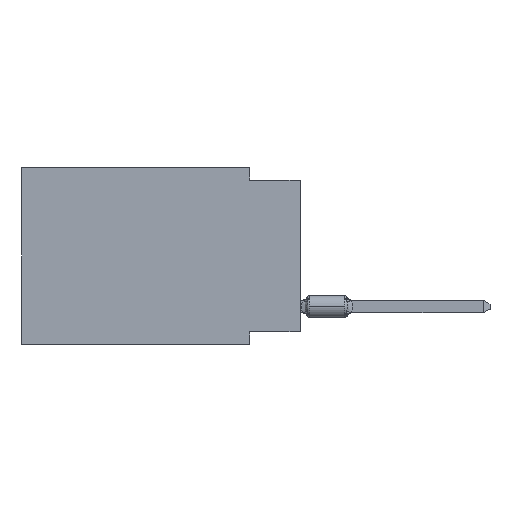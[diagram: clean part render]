
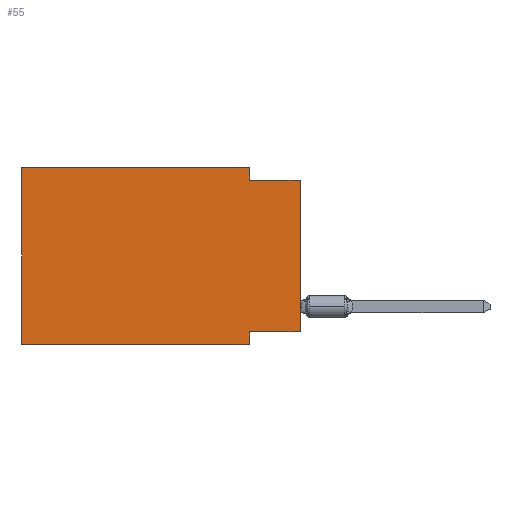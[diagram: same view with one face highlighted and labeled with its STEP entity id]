
A CAD part, left-side view. The second image highlights one B-rep face of the part: STEP entity #55.
In plain terms, the highlighted planar face has unit normal (-1, 0, 0).
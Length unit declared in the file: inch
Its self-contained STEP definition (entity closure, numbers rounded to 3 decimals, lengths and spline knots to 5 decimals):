
#55 = ADVANCED_FACE ( 'NONE', ( #3599 ), #19217, .F. ) ;
#631 = CARTESIAN_POINT ( 'NONE',  ( 0., 0., -0.025 ) ) ;
#648 = EDGE_CURVE ( 'NONE', #3919, #10364, #12601, .T. ) ;
#726 = CARTESIAN_POINT ( 'NONE',  ( 0., 0.1, -0.35 ) ) ;
#1348 = ORIENTED_EDGE ( 'NONE', *, *, #17111, .F. ) ;
#1421 = EDGE_CURVE ( 'NONE', #20242, #12905, #19560, .T. ) ;
#1776 = DIRECTION ( 'NONE',  ( 0., 0., -1. ) ) ;
#1805 = DIRECTION ( 'NONE',  ( 0., 0., 1. ) ) ;
#1895 = EDGE_CURVE ( 'NONE', #14072, #14090, #8160, .T. ) ;
#2567 = DIRECTION ( 'NONE',  ( 0., 1., 0. ) ) ;
#2668 = VECTOR ( 'NONE', #4640, 39.37008 ) ;
#2673 = VECTOR ( 'NONE', #1805, 39.37008 ) ;
#2706 = ORIENTED_EDGE ( 'NONE', *, *, #9855, .F. ) ;
#2844 = CARTESIAN_POINT ( 'NONE',  ( 0., 0.1, 0. ) ) ;
#2940 = DIRECTION ( 'NONE',  ( 0., 0., 1. ) ) ;
#3489 = CARTESIAN_POINT ( 'NONE',  ( 0., 0.1, 0. ) ) ;
#3599 = FACE_OUTER_BOUND ( 'NONE', #15670, .T. ) ;
#3919 = VERTEX_POINT ( 'NONE', #7776 ) ;
#4087 = CARTESIAN_POINT ( 'NONE',  ( 0., 0.1, -0.025 ) ) ;
#4640 = DIRECTION ( 'NONE',  ( 0., -1., 0. ) ) ;
#4720 = EDGE_CURVE ( 'NONE', #12905, #14090, #21774, .T. ) ;
#4862 = VECTOR ( 'NONE', #1776, 39.37008 ) ;
#5309 = LINE ( 'NONE', #15365, #2673 ) ;
#5687 = ORIENTED_EDGE ( 'NONE', *, *, #4720, .F. ) ;
#6359 = CARTESIAN_POINT ( 'NONE',  ( 0., 0., -0.025 ) ) ;
#7706 = VERTEX_POINT ( 'NONE', #4087 ) ;
#7766 = CARTESIAN_POINT ( 'NONE',  ( 0., 0., -0.325 ) ) ;
#7776 = CARTESIAN_POINT ( 'NONE',  ( 0., 0.55, 0. ) ) ;
#8050 = CARTESIAN_POINT ( 'NONE',  ( 0., 0.55, -0.35 ) ) ;
#8160 = LINE ( 'NONE', #13368, #8758 ) ;
#8254 = ORIENTED_EDGE ( 'NONE', *, *, #19964, .T. ) ;
#8422 = LINE ( 'NONE', #3489, #4862 ) ;
#8758 = VECTOR ( 'NONE', #15068, 39.37008 ) ;
#8788 = VECTOR ( 'NONE', #20188, 39.37008 ) ;
#9421 = ORIENTED_EDGE ( 'NONE', *, *, #20460, .F. ) ;
#9855 = EDGE_CURVE ( 'NONE', #7706, #18891, #12925, .T. ) ;
#10020 = LINE ( 'NONE', #21950, #14835 ) ;
#10288 = ORIENTED_EDGE ( 'NONE', *, *, #648, .F. ) ;
#10364 = VERTEX_POINT ( 'NONE', #2844 ) ;
#10466 = DIRECTION ( 'NONE',  ( 0., 0., -1. ) ) ;
#11010 = CARTESIAN_POINT ( 'NONE',  ( 0., 0.1, -0.35 ) ) ;
#11489 = VECTOR ( 'NONE', #2567, 39.37008 ) ;
#11862 = VECTOR ( 'NONE', #19756, 39.37008 ) ;
#12601 = LINE ( 'NONE', #14825, #2668 ) ;
#12905 = VERTEX_POINT ( 'NONE', #14359 ) ;
#12925 = LINE ( 'NONE', #6359, #8788 ) ;
#13310 = AXIS2_PLACEMENT_3D ( 'NONE', #20801, #20686, #10466 ) ;
#13368 = CARTESIAN_POINT ( 'NONE',  ( 0., 0.55, -0.35 ) ) ;
#14072 = VERTEX_POINT ( 'NONE', #8050 ) ;
#14090 = VERTEX_POINT ( 'NONE', #726 ) ;
#14359 = CARTESIAN_POINT ( 'NONE',  ( 0., 0.1, -0.325 ) ) ;
#14825 = CARTESIAN_POINT ( 'NONE',  ( 0., 0.55, 0. ) ) ;
#14835 = VECTOR ( 'NONE', #2940, 39.37008 ) ;
#15068 = DIRECTION ( 'NONE',  ( 0., -1., 0. ) ) ;
#15348 = ORIENTED_EDGE ( 'NONE', *, *, #1421, .F. ) ;
#15365 = CARTESIAN_POINT ( 'NONE',  ( 0., 0., 0. ) ) ;
#15670 = EDGE_LOOP ( 'NONE', ( #8254, #2706, #9421, #10288, #1348, #19715, #5687, #15348 ) ) ;
#16252 = CARTESIAN_POINT ( 'NONE',  ( 0., 0., -0.325 ) ) ;
#17111 = EDGE_CURVE ( 'NONE', #14072, #3919, #10020, .T. ) ;
#18891 = VERTEX_POINT ( 'NONE', #631 ) ;
#19217 = PLANE ( 'NONE',  #13310 ) ;
#19560 = LINE ( 'NONE', #16252, #11489 ) ;
#19715 = ORIENTED_EDGE ( 'NONE', *, *, #1895, .T. ) ;
#19756 = DIRECTION ( 'NONE',  ( 0., 0., -1. ) ) ;
#19964 = EDGE_CURVE ( 'NONE', #20242, #18891, #5309, .T. ) ;
#20188 = DIRECTION ( 'NONE',  ( 0., -1., 0. ) ) ;
#20242 = VERTEX_POINT ( 'NONE', #7766 ) ;
#20460 = EDGE_CURVE ( 'NONE', #10364, #7706, #8422, .T. ) ;
#20686 = DIRECTION ( 'NONE',  ( 1., 0., 0. ) ) ;
#20801 = CARTESIAN_POINT ( 'NONE',  ( 0., 0.55, 0. ) ) ;
#21774 = LINE ( 'NONE', #11010, #11862 ) ;
#21950 = CARTESIAN_POINT ( 'NONE',  ( 0., 0.55, 0. ) ) ;
